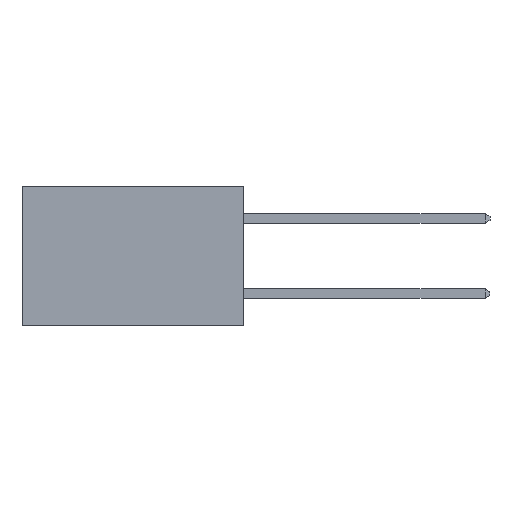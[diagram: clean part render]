
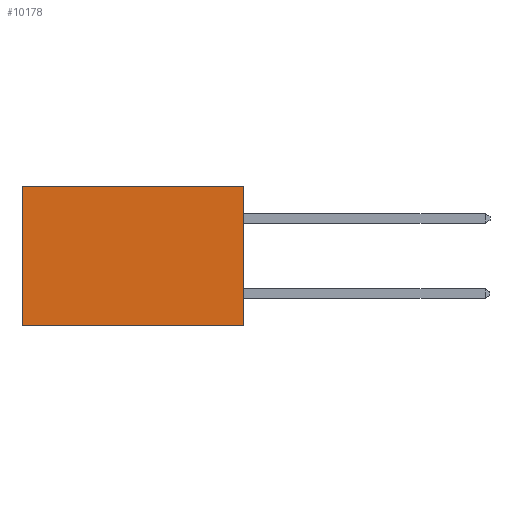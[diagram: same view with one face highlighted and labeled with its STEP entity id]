
A CAD part, left-side view. The second image highlights one B-rep face of the part: STEP entity #10178.
In plain terms, the highlighted planar face has unit normal (-1, 0, 0).
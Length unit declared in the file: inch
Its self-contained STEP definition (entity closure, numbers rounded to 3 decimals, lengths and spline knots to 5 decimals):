
#218 = VERTEX_POINT ( 'NONE', #4971 ) ;
#1102 = VECTOR ( 'NONE', #7458, 39.37008 ) ;
#1608 = LINE ( 'NONE', #9643, #4361 ) ;
#2188 = ORIENTED_EDGE ( 'NONE', *, *, #3339, .T. ) ;
#2734 = EDGE_LOOP ( 'NONE', ( #2188, #7534, #12047, #3305 ) ) ;
#2816 = FACE_OUTER_BOUND ( 'NONE', #2734, .T. ) ;
#3067 = VECTOR ( 'NONE', #5818, 39.37008 ) ;
#3263 = CARTESIAN_POINT ( 'NONE',  ( 0.277, 0., -0.37 ) ) ;
#3305 = ORIENTED_EDGE ( 'NONE', *, *, #7294, .T. ) ;
#3339 = EDGE_CURVE ( 'NONE', #5115, #218, #1608, .T. ) ;
#3391 = CARTESIAN_POINT ( 'NONE',  ( 0.277, 0.59, 0. ) ) ;
#4270 = DIRECTION ( 'NONE',  ( 0., 0., -1. ) ) ;
#4361 = VECTOR ( 'NONE', #9785, 39.37008 ) ;
#4563 = VERTEX_POINT ( 'NONE', #6786 ) ;
#4971 = CARTESIAN_POINT ( 'NONE',  ( 0.277, 0.59, -0.37 ) ) ;
#5037 = AXIS2_PLACEMENT_3D ( 'NONE', #3263, #10138, #4270 ) ;
#5115 = VERTEX_POINT ( 'NONE', #3391 ) ;
#5732 = LINE ( 'NONE', #6315, #3067 ) ;
#5818 = DIRECTION ( 'NONE',  ( 0., 1., 0. ) ) ;
#5904 = LINE ( 'NONE', #9408, #1102 ) ;
#6315 = CARTESIAN_POINT ( 'NONE',  ( 0.277, 0., 0. ) ) ;
#6786 = CARTESIAN_POINT ( 'NONE',  ( 0.277, 0., -0.37 ) ) ;
#7294 = EDGE_CURVE ( 'NONE', #8411, #5115, #5732, .T. ) ;
#7458 = DIRECTION ( 'NONE',  ( 0., 0., -1. ) ) ;
#7534 = ORIENTED_EDGE ( 'NONE', *, *, #10478, .F. ) ;
#7645 = DIRECTION ( 'NONE',  ( 0., 1., 0. ) ) ;
#8222 = PLANE ( 'NONE',  #5037 ) ;
#8411 = VERTEX_POINT ( 'NONE', #11213 ) ;
#8623 = CARTESIAN_POINT ( 'NONE',  ( 0.277, 0., -0.37 ) ) ;
#9408 = CARTESIAN_POINT ( 'NONE',  ( 0.277, 0., -0.37 ) ) ;
#9643 = CARTESIAN_POINT ( 'NONE',  ( 0.277, 0.59, -0.37 ) ) ;
#9785 = DIRECTION ( 'NONE',  ( 0., 0., -1. ) ) ;
#10138 = DIRECTION ( 'NONE',  ( 1., 0., 0. ) ) ;
#10178 = ADVANCED_FACE ( 'NONE', ( #2816 ), #8222, .F. ) ;
#10216 = LINE ( 'NONE', #8623, #12441 ) ;
#10478 = EDGE_CURVE ( 'NONE', #4563, #218, #10216, .T. ) ;
#11213 = CARTESIAN_POINT ( 'NONE',  ( 0.277, 0., 0. ) ) ;
#12047 = ORIENTED_EDGE ( 'NONE', *, *, #12161, .F. ) ;
#12161 = EDGE_CURVE ( 'NONE', #8411, #4563, #5904, .T. ) ;
#12441 = VECTOR ( 'NONE', #7645, 39.37008 ) ;
